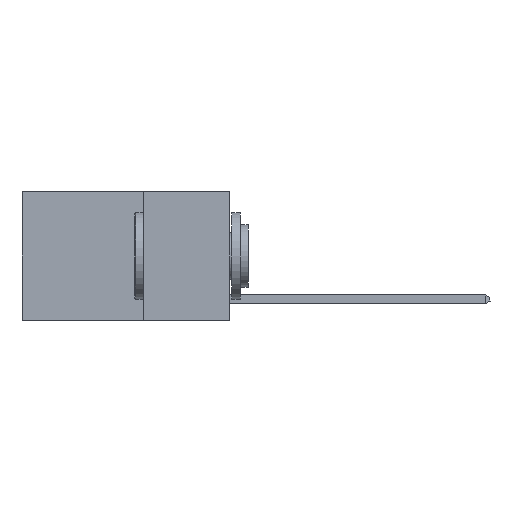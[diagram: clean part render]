
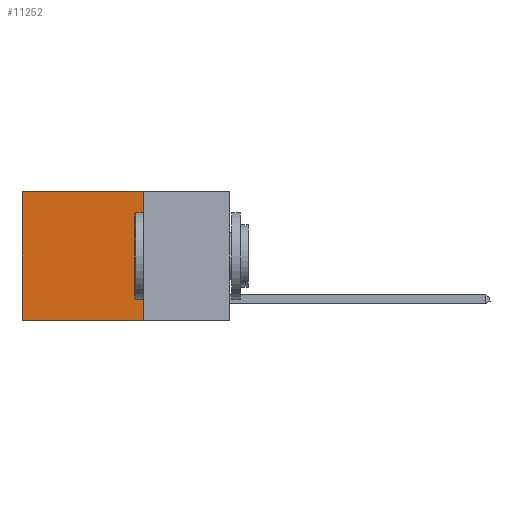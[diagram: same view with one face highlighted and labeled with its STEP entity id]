
A CAD part, left-side view. The second image highlights one B-rep face of the part: STEP entity #11252.
In plain terms, the highlighted planar face has unit normal (-1, 0, 0).
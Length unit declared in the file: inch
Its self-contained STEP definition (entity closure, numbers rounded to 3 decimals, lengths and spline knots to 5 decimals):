
#657 = CARTESIAN_POINT ( 'NONE',  ( 0.2625, 0.6, 0. ) ) ;
#809 = VERTEX_POINT ( 'NONE', #4932 ) ;
#1900 = LINE ( 'NONE', #2933, #13783 ) ;
#2310 = CARTESIAN_POINT ( 'NONE',  ( 0.2625, 0.25, 0. ) ) ;
#2311 = LINE ( 'NONE', #4598, #4393 ) ;
#2704 = LINE ( 'NONE', #657, #4675 ) ;
#2928 = EDGE_LOOP ( 'NONE', ( #11310, #7774, #6318, #5263 ) ) ;
#2933 = CARTESIAN_POINT ( 'NONE',  ( 0.2625, 0.25, 0. ) ) ;
#3084 = VERTEX_POINT ( 'NONE', #11067 ) ;
#3140 = EDGE_CURVE ( 'NONE', #6479, #3084, #2311, .T. ) ;
#3245 = DIRECTION ( 'NONE',  ( 0., 0., -1. ) ) ;
#4393 = VECTOR ( 'NONE', #9094, 39.37008 ) ;
#4598 = CARTESIAN_POINT ( 'NONE',  ( 0.2625, 0.25, 0. ) ) ;
#4675 = VECTOR ( 'NONE', #5163, 39.37008 ) ;
#4745 = CARTESIAN_POINT ( 'NONE',  ( 0.2625, 0.25, 0. ) ) ;
#4932 = CARTESIAN_POINT ( 'NONE',  ( 0.2625, 0.6, -0.37 ) ) ;
#5163 = DIRECTION ( 'NONE',  ( 0., 0., -1. ) ) ;
#5236 = DIRECTION ( 'NONE',  ( 0., 1., 0. ) ) ;
#5263 = ORIENTED_EDGE ( 'NONE', *, *, #12031, .T. ) ;
#6318 = ORIENTED_EDGE ( 'NONE', *, *, #3140, .F. ) ;
#6392 = CARTESIAN_POINT ( 'NONE',  ( 0.2625, 0.6, 0. ) ) ;
#6479 = VERTEX_POINT ( 'NONE', #2310 ) ;
#6495 = AXIS2_PLACEMENT_3D ( 'NONE', #4745, #9230, #3245 ) ;
#6870 = VERTEX_POINT ( 'NONE', #6392 ) ;
#7591 = LINE ( 'NONE', #10942, #7952 ) ;
#7751 = EDGE_CURVE ( 'NONE', #3084, #809, #7591, .T. ) ;
#7774 = ORIENTED_EDGE ( 'NONE', *, *, #7751, .F. ) ;
#7952 = VECTOR ( 'NONE', #5236, 39.37008 ) ;
#9094 = DIRECTION ( 'NONE',  ( 0., 0., -1. ) ) ;
#9230 = DIRECTION ( 'NONE',  ( 1., 0., 0. ) ) ;
#9783 = DIRECTION ( 'NONE',  ( 0., 1., 0. ) ) ;
#10942 = CARTESIAN_POINT ( 'NONE',  ( 0.2625, 0.25, -0.37 ) ) ;
#11067 = CARTESIAN_POINT ( 'NONE',  ( 0.2625, 0.25, -0.37 ) ) ;
#11124 = PLANE ( 'NONE',  #6495 ) ;
#11252 = ADVANCED_FACE ( 'NONE', ( #11424 ), #11124, .F. ) ;
#11310 = ORIENTED_EDGE ( 'NONE', *, *, #13589, .T. ) ;
#11424 = FACE_OUTER_BOUND ( 'NONE', #2928, .T. ) ;
#12031 = EDGE_CURVE ( 'NONE', #6479, #6870, #1900, .T. ) ;
#13589 = EDGE_CURVE ( 'NONE', #6870, #809, #2704, .T. ) ;
#13783 = VECTOR ( 'NONE', #9783, 39.37008 ) ;
